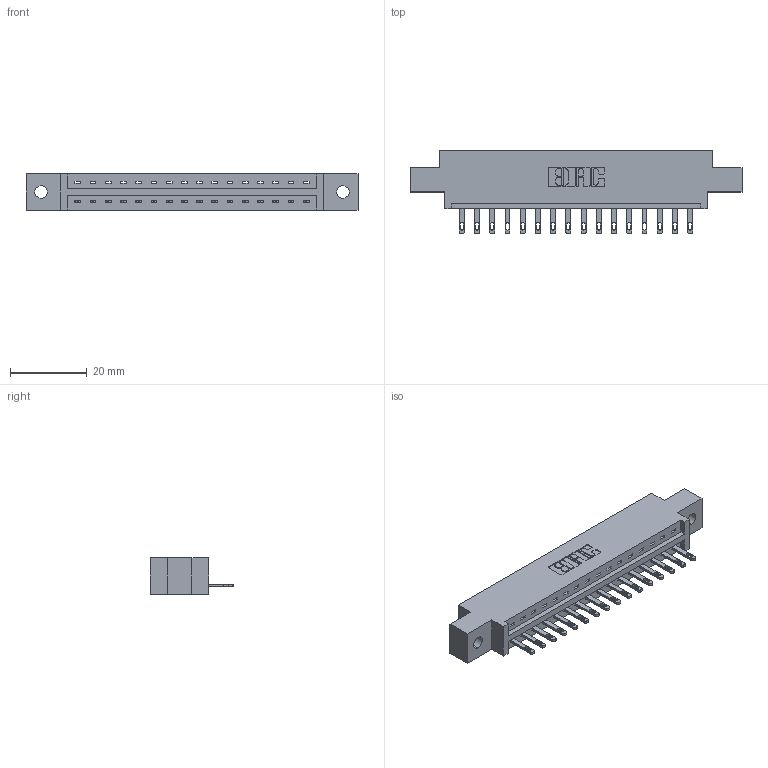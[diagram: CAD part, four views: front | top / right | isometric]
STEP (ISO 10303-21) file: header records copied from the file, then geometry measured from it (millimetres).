
FILE_DESCRIPTION (( 'STEP AP203' ), '1' );
FILE_NAME ('887-016-500-602.STEP', '2020-09-20T17:16:46', ( '' ), ( '' ), 'SwSTEP 2.0', 'SolidWorks 2020', '' );
FILE_SCHEMA (( 'CONFIG_CONTROL_DESIGN' ));
Length unit declared in the file: inch
Products named in the file (3): 837 Part_0.170 Offset - 0.128 Dia; 345-292-001_345-293-100; 887-016-500-602
Assembly tree (17 placements, depth 2):
  887-016-500-602
    837 Part_0.170 Offset - 0.128 Dia
    345-292-001_345-293-100  x16
Bounding box: 86.41 x 21.85 x 9.4 mm (x, y, z)
Volume: 8511.3 mm3; surface area: 8514.8 mm2
Topology: 17 solids, 17 shells, 1046 faces, 3203 edges, 2134 vertices
Faces by surface type: plane 714, cylinder 332
Entity records: 15321 total; most frequent: CARTESIAN_POINT 2674, ORIENTED_EDGE 2626, DIRECTION 2305, EDGE_CURVE 1313, LINE 1181, VECTOR 1181, VERTEX_POINT 874, AXIS2_PLACEMENT_3D 562
